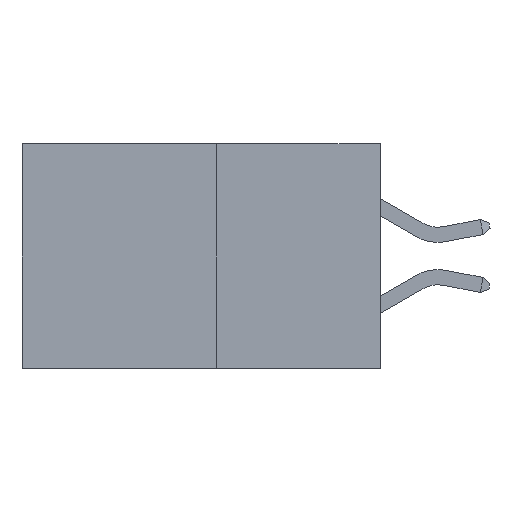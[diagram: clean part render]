
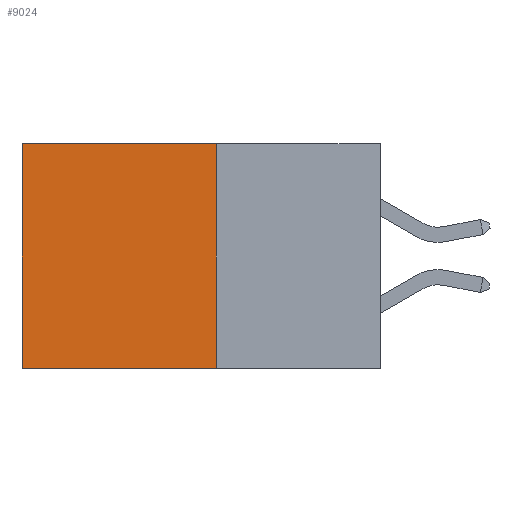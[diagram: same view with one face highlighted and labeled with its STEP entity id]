
A CAD part, left-side view. The second image highlights one B-rep face of the part: STEP entity #9024.
In plain terms, the highlighted planar face has unit normal (-1, 0, 0).
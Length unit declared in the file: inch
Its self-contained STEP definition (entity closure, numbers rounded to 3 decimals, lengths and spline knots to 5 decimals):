
#164 = CARTESIAN_POINT ( 'NONE',  ( 0.277, 0.59, -0.37 ) ) ;
#738 = VECTOR ( 'NONE', #8382, 39.37008 ) ;
#2332 = ORIENTED_EDGE ( 'NONE', *, *, #6946, .F. ) ;
#2790 = CARTESIAN_POINT ( 'NONE',  ( 0.277, 0.27, 0. ) ) ;
#3515 = FACE_OUTER_BOUND ( 'NONE', #6230, .T. ) ;
#4116 = VECTOR ( 'NONE', #4826, 39.37008 ) ;
#4532 = DIRECTION ( 'NONE',  ( 0., 0., -1. ) ) ;
#4826 = DIRECTION ( 'NONE',  ( 0., 0., -1. ) ) ;
#4919 = ORIENTED_EDGE ( 'NONE', *, *, #9840, .T. ) ;
#5282 = AXIS2_PLACEMENT_3D ( 'NONE', #9567, #12170, #4532 ) ;
#5459 = EDGE_CURVE ( 'NONE', #14763, #9267, #15797, .T. ) ;
#5687 = EDGE_CURVE ( 'NONE', #14763, #14871, #12771, .T. ) ;
#5857 = VECTOR ( 'NONE', #9191, 39.37008 ) ;
#6055 = VECTOR ( 'NONE', #14317, 39.37008 ) ;
#6163 = ORIENTED_EDGE ( 'NONE', *, *, #5459, .F. ) ;
#6230 = EDGE_LOOP ( 'NONE', ( #4919, #2332, #6163, #13638 ) ) ;
#6837 = CARTESIAN_POINT ( 'NONE',  ( 0.277, 0.59, 0. ) ) ;
#6946 = EDGE_CURVE ( 'NONE', #9267, #11764, #7603, .T. ) ;
#7258 = CARTESIAN_POINT ( 'NONE',  ( 0.277, 0.27, 0. ) ) ;
#7527 = LINE ( 'NONE', #8659, #4116 ) ;
#7603 = LINE ( 'NONE', #14654, #738 ) ;
#8382 = DIRECTION ( 'NONE',  ( 0., 1., 0. ) ) ;
#8659 = CARTESIAN_POINT ( 'NONE',  ( 0.277, 0.59, -0.37 ) ) ;
#8838 = CARTESIAN_POINT ( 'NONE',  ( 0.277, 0.27, -0.37 ) ) ;
#9024 = ADVANCED_FACE ( 'NONE', ( #3515 ), #10906, .F. ) ;
#9191 = DIRECTION ( 'NONE',  ( 0., 0., -1. ) ) ;
#9267 = VERTEX_POINT ( 'NONE', #8838 ) ;
#9442 = CARTESIAN_POINT ( 'NONE',  ( 0.277, 0.27, -0.37 ) ) ;
#9567 = CARTESIAN_POINT ( 'NONE',  ( 0.277, 0.27, -0.37 ) ) ;
#9840 = EDGE_CURVE ( 'NONE', #14871, #11764, #7527, .T. ) ;
#10906 = PLANE ( 'NONE',  #5282 ) ;
#11764 = VERTEX_POINT ( 'NONE', #164 ) ;
#12170 = DIRECTION ( 'NONE',  ( 1., 0., 0. ) ) ;
#12771 = LINE ( 'NONE', #7258, #6055 ) ;
#13638 = ORIENTED_EDGE ( 'NONE', *, *, #5687, .T. ) ;
#14317 = DIRECTION ( 'NONE',  ( 0., 1., 0. ) ) ;
#14654 = CARTESIAN_POINT ( 'NONE',  ( 0.277, 0.27, -0.37 ) ) ;
#14763 = VERTEX_POINT ( 'NONE', #2790 ) ;
#14871 = VERTEX_POINT ( 'NONE', #6837 ) ;
#15797 = LINE ( 'NONE', #9442, #5857 ) ;
